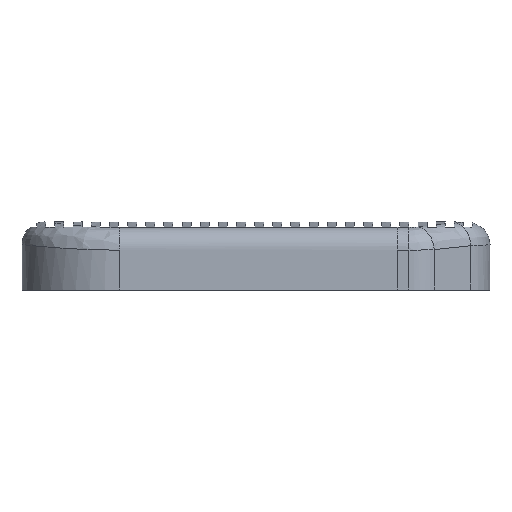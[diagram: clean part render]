
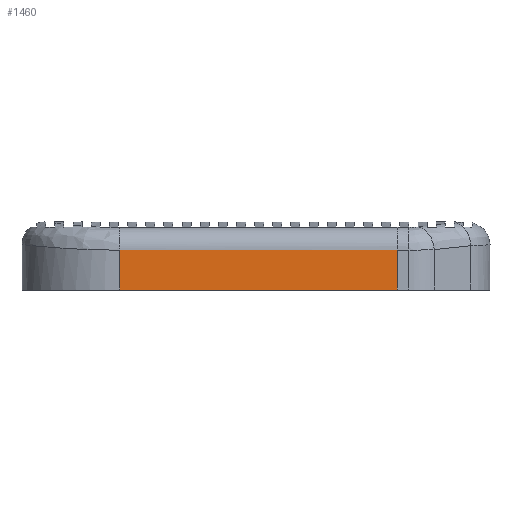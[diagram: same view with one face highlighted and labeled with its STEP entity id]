
A CAD part, left-side view. The second image highlights one B-rep face of the part: STEP entity #1460.
In plain terms, the highlighted planar face has unit normal (-1, -0.014, 0).
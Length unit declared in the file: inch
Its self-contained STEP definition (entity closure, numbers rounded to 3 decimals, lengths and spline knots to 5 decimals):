
#85 = ORIENTED_EDGE ( 'NONE', *, *, #1729, .T. ) ;
#410 = VECTOR ( 'NONE', #4930, 39.37008 ) ;
#821 = DIRECTION ( 'NONE',  ( 0., 0., -1. ) ) ;
#840 = ORIENTED_EDGE ( 'NONE', *, *, #4040, .T. ) ;
#953 = EDGE_LOOP ( 'NONE', ( #1197, #4883, #5830, #840, #85 ) ) ;
#1022 = LINE ( 'NONE', #5557, #4865 ) ;
#1027 = LINE ( 'NONE', #4353, #6029 ) ;
#1197 = ORIENTED_EDGE ( 'NONE', *, *, #3181, .F. ) ;
#1460 = ADVANCED_FACE ( 'NONE', ( #3687 ), #3995, .F. ) ;
#1493 = DIRECTION ( 'NONE',  ( -0.014, 1., 0. ) ) ;
#1546 = CARTESIAN_POINT ( 'NONE',  ( -1.41989, -1.15531, -0.07865 ) ) ;
#1562 = EDGE_CURVE ( 'NONE', #3952, #5761, #1027, .T. ) ;
#1729 = EDGE_CURVE ( 'NONE', #4994, #6395, #4395, .T. ) ;
#1971 = CARTESIAN_POINT ( 'NONE',  ( -1.46391, 1.89855, 0.31505 ) ) ;
#2527 = VECTOR ( 'NONE', #821, 39.37008 ) ;
#2999 = VECTOR ( 'NONE', #5242, 39.37008 ) ;
#3181 = EDGE_CURVE ( 'NONE', #3727, #6395, #5174, .T. ) ;
#3274 = EDGE_CURVE ( 'NONE', #3727, #3952, #1022, .T. ) ;
#3687 = FACE_OUTER_BOUND ( 'NONE', #953, .T. ) ;
#3727 = VERTEX_POINT ( 'NONE', #5660 ) ;
#3891 = CARTESIAN_POINT ( 'NONE',  ( -1.46391, 1.89855, -0.07865 ) ) ;
#3952 = VERTEX_POINT ( 'NONE', #6190 ) ;
#3995 = PLANE ( 'NONE',  #5519 ) ;
#4040 = EDGE_CURVE ( 'NONE', #5761, #4994, #5810, .T. ) ;
#4353 = CARTESIAN_POINT ( 'NONE',  ( -1.46391, 1.89855, 0.36146 ) ) ;
#4395 = LINE ( 'NONE', #3891, #410 ) ;
#4494 = DIRECTION ( 'NONE',  ( 1., 0.014, 0. ) ) ;
#4839 = CARTESIAN_POINT ( 'NONE',  ( -1.41989, -1.15531, 0.31505 ) ) ;
#4860 = DIRECTION ( 'NONE',  ( -0.014, 1., 0. ) ) ;
#4865 = VECTOR ( 'NONE', #6043, 39.37008 ) ;
#4883 = ORIENTED_EDGE ( 'NONE', *, *, #3274, .T. ) ;
#4930 = DIRECTION ( 'NONE',  ( 0.014, -1., 0. ) ) ;
#4952 = CARTESIAN_POINT ( 'NONE',  ( -1.46391, 1.89855, -0.07865 ) ) ;
#4994 = VERTEX_POINT ( 'NONE', #4952 ) ;
#5174 = LINE ( 'NONE', #4839, #2527 ) ;
#5242 = DIRECTION ( 'NONE',  ( 0., 0., -1. ) ) ;
#5519 = AXIS2_PLACEMENT_3D ( 'NONE', #1971, #4494, #1493 ) ;
#5557 = CARTESIAN_POINT ( 'NONE',  ( -1.41989, -1.15531, 0.36146 ) ) ;
#5622 = CARTESIAN_POINT ( 'NONE',  ( -1.46391, 1.89855, 0.36146 ) ) ;
#5660 = CARTESIAN_POINT ( 'NONE',  ( -1.41989, -1.15531, 0.36146 ) ) ;
#5761 = VERTEX_POINT ( 'NONE', #5622 ) ;
#5810 = LINE ( 'NONE', #6239, #2999 ) ;
#5830 = ORIENTED_EDGE ( 'NONE', *, *, #1562, .T. ) ;
#6029 = VECTOR ( 'NONE', #4860, 39.37008 ) ;
#6043 = DIRECTION ( 'NONE',  ( 0., 0., 1. ) ) ;
#6190 = CARTESIAN_POINT ( 'NONE',  ( -1.41989, -1.15531, 0.36146 ) ) ;
#6239 = CARTESIAN_POINT ( 'NONE',  ( -1.46391, 1.89855, 0.31505 ) ) ;
#6395 = VERTEX_POINT ( 'NONE', #1546 ) ;
